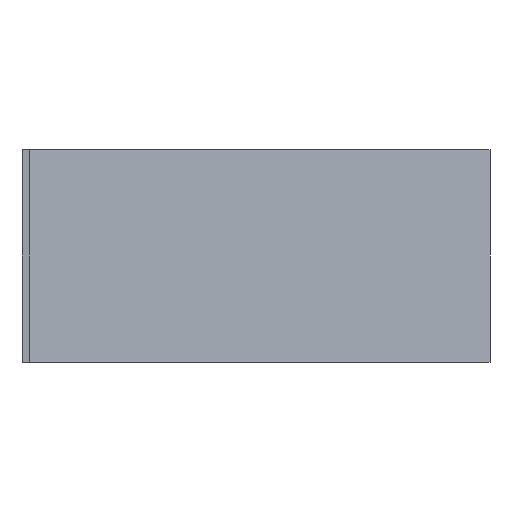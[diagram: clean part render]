
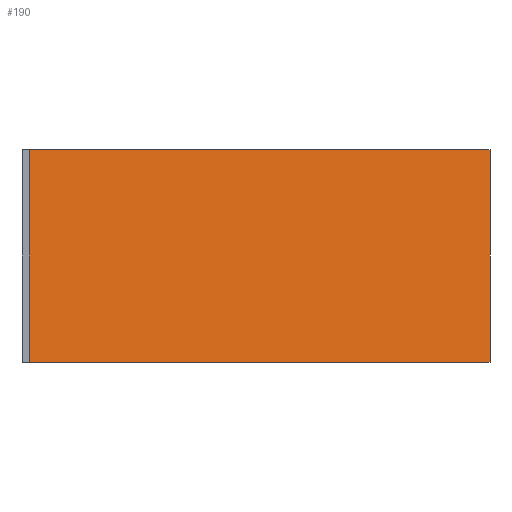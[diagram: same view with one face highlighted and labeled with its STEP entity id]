
A CAD part, front view. The second image highlights one B-rep face of the part: STEP entity #190.
In plain terms, the highlighted planar face has unit normal (0.174, -0.985, 0).
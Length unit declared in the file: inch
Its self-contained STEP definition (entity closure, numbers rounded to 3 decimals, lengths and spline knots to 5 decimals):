
#7 = VERTEX_POINT ( 'NONE', #168 ) ;
#14 = VERTEX_POINT ( 'NONE', #23 ) ;
#23 = CARTESIAN_POINT ( 'NONE',  ( 0.02, 1.98353, 0. ) ) ;
#24 = CARTESIAN_POINT ( 'NONE',  ( 1.3, 2.20923, 0.59 ) ) ;
#25 = DIRECTION ( 'NONE',  ( 0., 0., 1. ) ) ;
#42 = PLANE ( 'NONE',  #247 ) ;
#53 = EDGE_LOOP ( 'NONE', ( #91, #188, #70, #114 ) ) ;
#70 = ORIENTED_EDGE ( 'NONE', *, *, #159, .F. ) ;
#77 = CARTESIAN_POINT ( 'NONE',  ( 1.3, 2.20923, 0. ) ) ;
#79 = VECTOR ( 'NONE', #207, 39.37008 ) ;
#83 = DIRECTION ( 'NONE',  ( 0.985, 0.174, 0. ) ) ;
#91 = ORIENTED_EDGE ( 'NONE', *, *, #117, .T. ) ;
#114 = ORIENTED_EDGE ( 'NONE', *, *, #232, .T. ) ;
#117 = EDGE_CURVE ( 'NONE', #223, #122, #266, .T. ) ;
#122 = VERTEX_POINT ( 'NONE', #24 ) ;
#130 = FACE_OUTER_BOUND ( 'NONE', #53, .T. ) ;
#138 = LINE ( 'NONE', #227, #79 ) ;
#140 = EDGE_CURVE ( 'NONE', #7, #122, #196, .T. ) ;
#143 = VECTOR ( 'NONE', #267, 39.37008 ) ;
#150 = CARTESIAN_POINT ( 'NONE',  ( 0.02, 1.98353, 0. ) ) ;
#152 = DIRECTION ( 'NONE',  ( 0.985, 0.174, 0. ) ) ;
#158 = VECTOR ( 'NONE', #25, 39.37008 ) ;
#159 = EDGE_CURVE ( 'NONE', #14, #7, #274, .T. ) ;
#163 = DIRECTION ( 'NONE',  ( 0.174, -0.985, 0. ) ) ;
#168 = CARTESIAN_POINT ( 'NONE',  ( 0.02, 1.98353, 0.59 ) ) ;
#188 = ORIENTED_EDGE ( 'NONE', *, *, #140, .F. ) ;
#190 = ADVANCED_FACE ( 'NONE', ( #130 ), #42, .T. ) ;
#196 = LINE ( 'NONE', #240, #212 ) ;
#207 = DIRECTION ( 'NONE',  ( 0.985, 0.174, 0. ) ) ;
#212 = VECTOR ( 'NONE', #152, 39.37008 ) ;
#223 = VERTEX_POINT ( 'NONE', #77 ) ;
#227 = CARTESIAN_POINT ( 'NONE',  ( 0.02, 1.98353, 0. ) ) ;
#232 = EDGE_CURVE ( 'NONE', #14, #223, #138, .T. ) ;
#239 = CARTESIAN_POINT ( 'NONE',  ( 1.3, 2.20923, 0. ) ) ;
#240 = CARTESIAN_POINT ( 'NONE',  ( 0.02, 1.98353, 0.59 ) ) ;
#247 = AXIS2_PLACEMENT_3D ( 'NONE', #260, #163, #83 ) ;
#260 = CARTESIAN_POINT ( 'NONE',  ( 0.02, 1.98353, 0. ) ) ;
#266 = LINE ( 'NONE', #239, #158 ) ;
#267 = DIRECTION ( 'NONE',  ( 0., 0., 1. ) ) ;
#274 = LINE ( 'NONE', #150, #143 ) ;
